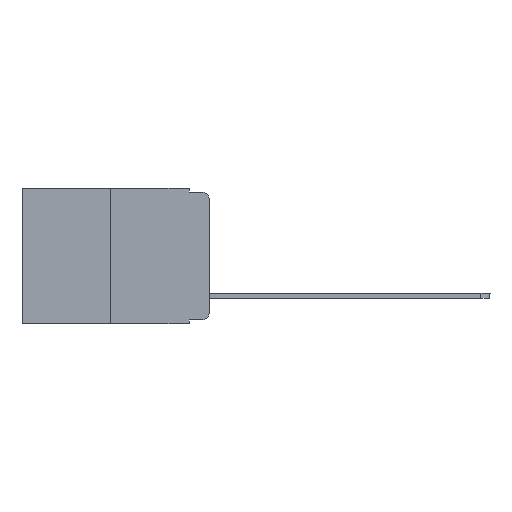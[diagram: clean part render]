
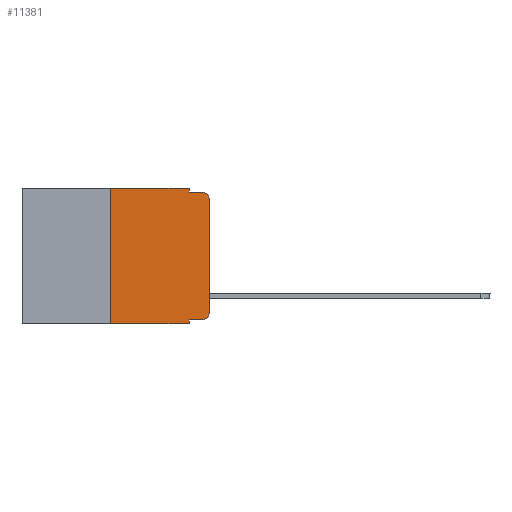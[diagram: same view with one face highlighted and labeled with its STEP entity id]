
A CAD part, left-side view. The second image highlights one B-rep face of the part: STEP entity #11381.
In plain terms, the highlighted planar face has unit normal (-1, 0, 0).
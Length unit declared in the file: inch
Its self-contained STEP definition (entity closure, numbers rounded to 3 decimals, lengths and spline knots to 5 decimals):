
#33 = DIRECTION ( 'NONE',  ( 0., 0., 1. ) ) ;
#134 = DIRECTION ( 'NONE',  ( 0., 0., -1. ) ) ;
#201 = VECTOR ( 'NONE', #33, 39.37008 ) ;
#252 = CARTESIAN_POINT ( 'NONE',  ( 0., 0.02, -0.03 ) ) ;
#307 = DIRECTION ( 'NONE',  ( 0., -1., 0. ) ) ;
#321 = CARTESIAN_POINT ( 'NONE',  ( 0., 0.25, 0. ) ) ;
#689 = VERTEX_POINT ( 'NONE', #2291 ) ;
#949 = ORIENTED_EDGE ( 'NONE', *, *, #9207, .T. ) ;
#989 = EDGE_CURVE ( 'NONE', #4083, #3147, #9395, .T. ) ;
#1041 = DIRECTION ( 'NONE',  ( 0., -1., 0. ) ) ;
#1137 = LINE ( 'NONE', #1258, #2826 ) ;
#1258 = CARTESIAN_POINT ( 'NONE',  ( 0., 0.473, 0. ) ) ;
#1472 = ORIENTED_EDGE ( 'NONE', *, *, #6206, .F. ) ;
#1685 = LINE ( 'NONE', #6365, #6930 ) ;
#1933 = ORIENTED_EDGE ( 'NONE', *, *, #5357, .T. ) ;
#2061 = ORIENTED_EDGE ( 'NONE', *, *, #2778, .F. ) ;
#2105 = VERTEX_POINT ( 'NONE', #3823 ) ;
#2291 = CARTESIAN_POINT ( 'NONE',  ( 0., 0.25, -0.343 ) ) ;
#2496 = LINE ( 'NONE', #9907, #5778 ) ;
#2778 = EDGE_CURVE ( 'NONE', #4284, #3147, #5721, .T. ) ;
#2826 = VECTOR ( 'NONE', #3898, 39.37008 ) ;
#2900 = EDGE_CURVE ( 'NONE', #689, #8024, #4707, .T. ) ;
#3147 = VERTEX_POINT ( 'NONE', #4614 ) ;
#3199 = VECTOR ( 'NONE', #11755, 39.37008 ) ;
#3416 = CARTESIAN_POINT ( 'NONE',  ( 0., 0.051, -0.333 ) ) ;
#3823 = CARTESIAN_POINT ( 'NONE',  ( 0., 0., -0.313 ) ) ;
#3898 = DIRECTION ( 'NONE',  ( 0., -1., 0. ) ) ;
#3972 = LINE ( 'NONE', #11332, #5767 ) ;
#3987 = AXIS2_PLACEMENT_3D ( 'NONE', #11743, #4213, #4320 ) ;
#4083 = VERTEX_POINT ( 'NONE', #10794 ) ;
#4213 = DIRECTION ( 'NONE',  ( -1., 0., 0. ) ) ;
#4284 = VERTEX_POINT ( 'NONE', #6413 ) ;
#4320 = DIRECTION ( 'NONE',  ( 0., 0., -1. ) ) ;
#4406 = LINE ( 'NONE', #3416, #3199 ) ;
#4503 = EDGE_CURVE ( 'NONE', #689, #12078, #11711, .T. ) ;
#4614 = CARTESIAN_POINT ( 'NONE',  ( 0., 0.02, -0.01 ) ) ;
#4624 = ORIENTED_EDGE ( 'NONE', *, *, #2900, .F. ) ;
#4707 = LINE ( 'NONE', #8476, #201 ) ;
#4933 = CARTESIAN_POINT ( 'NONE',  ( 0., 0.473, -0.343 ) ) ;
#5104 = VERTEX_POINT ( 'NONE', #5514 ) ;
#5357 = EDGE_CURVE ( 'NONE', #5104, #2105, #6534, .T. ) ;
#5514 = CARTESIAN_POINT ( 'NONE',  ( 0., 0.02, -0.333 ) ) ;
#5721 = LINE ( 'NONE', #6709, #10192 ) ;
#5767 = VECTOR ( 'NONE', #7745, 39.37008 ) ;
#5778 = VECTOR ( 'NONE', #9036, 39.37008 ) ;
#6206 = EDGE_CURVE ( 'NONE', #12106, #12078, #2496, .T. ) ;
#6365 = CARTESIAN_POINT ( 'NONE',  ( 0., 0., 0. ) ) ;
#6413 = CARTESIAN_POINT ( 'NONE',  ( 0., 0.051, -0.01 ) ) ;
#6534 = CIRCLE ( 'NONE', #3987, 0.02 ) ;
#6608 = DIRECTION ( 'NONE',  ( 0., 0., 1. ) ) ;
#6709 = CARTESIAN_POINT ( 'NONE',  ( 0., 0.051, -0.01 ) ) ;
#6854 = ORIENTED_EDGE ( 'NONE', *, *, #4503, .T. ) ;
#6930 = VECTOR ( 'NONE', #6608, 39.37008 ) ;
#7075 = VERTEX_POINT ( 'NONE', #10338 ) ;
#7292 = EDGE_CURVE ( 'NONE', #12106, #5104, #4406, .T. ) ;
#7309 = DIRECTION ( 'NONE',  ( 0., 0., -1. ) ) ;
#7613 = ORIENTED_EDGE ( 'NONE', *, *, #10670, .F. ) ;
#7745 = DIRECTION ( 'NONE',  ( 0., 0., -1. ) ) ;
#7838 = DIRECTION ( 'NONE',  ( -1., 0., 0. ) ) ;
#8024 = VERTEX_POINT ( 'NONE', #321 ) ;
#8028 = AXIS2_PLACEMENT_3D ( 'NONE', #252, #7838, #134 ) ;
#8059 = FACE_OUTER_BOUND ( 'NONE', #11775, .T. ) ;
#8476 = CARTESIAN_POINT ( 'NONE',  ( 0., 0.25, 0. ) ) ;
#8519 = CARTESIAN_POINT ( 'NONE',  ( 0., 0.051, -0.333 ) ) ;
#8644 = CARTESIAN_POINT ( 'NONE',  ( 0., 0.051, -0.343 ) ) ;
#9036 = DIRECTION ( 'NONE',  ( 0., 0., -1. ) ) ;
#9157 = DIRECTION ( 'NONE',  ( 1., 0., 0. ) ) ;
#9207 = EDGE_CURVE ( 'NONE', #2105, #4083, #1685, .T. ) ;
#9333 = ORIENTED_EDGE ( 'NONE', *, *, #989, .T. ) ;
#9395 = CIRCLE ( 'NONE', #8028, 0.02 ) ;
#9883 = VECTOR ( 'NONE', #307, 39.37008 ) ;
#9907 = CARTESIAN_POINT ( 'NONE',  ( 0., 0.051, 0. ) ) ;
#10192 = VECTOR ( 'NONE', #1041, 39.37008 ) ;
#10311 = AXIS2_PLACEMENT_3D ( 'NONE', #11872, #9157, #7309 ) ;
#10338 = CARTESIAN_POINT ( 'NONE',  ( 0., 0.051, 0. ) ) ;
#10647 = ORIENTED_EDGE ( 'NONE', *, *, #11737, .F. ) ;
#10670 = EDGE_CURVE ( 'NONE', #7075, #4284, #3972, .T. ) ;
#10794 = CARTESIAN_POINT ( 'NONE',  ( 0., 0., -0.03 ) ) ;
#10817 = PLANE ( 'NONE',  #10311 ) ;
#10961 = ORIENTED_EDGE ( 'NONE', *, *, #7292, .T. ) ;
#11332 = CARTESIAN_POINT ( 'NONE',  ( 0., 0.051, 0. ) ) ;
#11381 = ADVANCED_FACE ( 'NONE', ( #8059 ), #10817, .F. ) ;
#11711 = LINE ( 'NONE', #4933, #9883 ) ;
#11737 = EDGE_CURVE ( 'NONE', #8024, #7075, #1137, .T. ) ;
#11743 = CARTESIAN_POINT ( 'NONE',  ( 0., 0.02, -0.313 ) ) ;
#11755 = DIRECTION ( 'NONE',  ( 0., -1., 0. ) ) ;
#11775 = EDGE_LOOP ( 'NONE', ( #949, #9333, #2061, #7613, #10647, #4624, #6854, #1472, #10961, #1933 ) ) ;
#11872 = CARTESIAN_POINT ( 'NONE',  ( 0., 0.473, 0. ) ) ;
#12078 = VERTEX_POINT ( 'NONE', #8644 ) ;
#12106 = VERTEX_POINT ( 'NONE', #8519 ) ;
